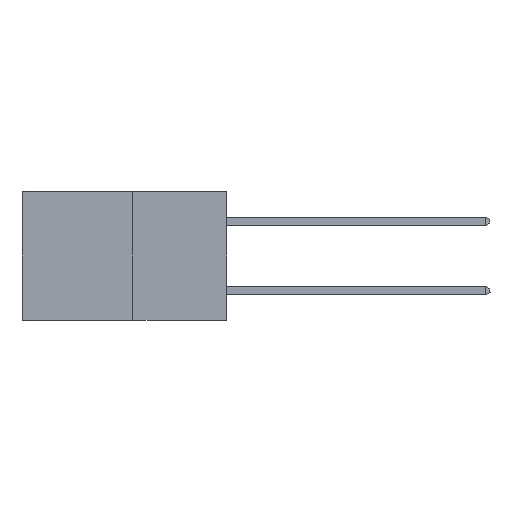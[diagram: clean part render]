
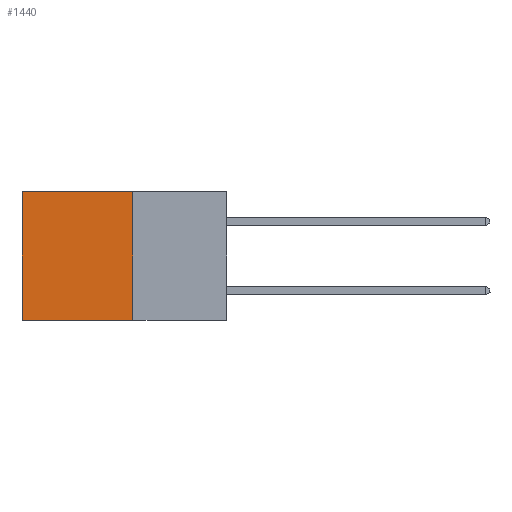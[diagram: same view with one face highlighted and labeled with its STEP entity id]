
A CAD part, left-side view. The second image highlights one B-rep face of the part: STEP entity #1440.
In plain terms, the highlighted planar face has unit normal (-1, 0, 0).
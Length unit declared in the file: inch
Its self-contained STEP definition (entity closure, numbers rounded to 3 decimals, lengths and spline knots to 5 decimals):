
#125 = ORIENTED_EDGE ( 'NONE', *, *, #4721, .T. ) ;
#273 = ORIENTED_EDGE ( 'NONE', *, *, #5878, .F. ) ;
#438 = VERTEX_POINT ( 'NONE', #6912 ) ;
#564 = DIRECTION ( 'NONE',  ( 0., 1., 0. ) ) ;
#742 = CARTESIAN_POINT ( 'NONE',  ( 0.277, 0.27, -0.37 ) ) ;
#805 = LINE ( 'NONE', #8846, #3185 ) ;
#1440 = ADVANCED_FACE ( 'NONE', ( #3838 ), #8367, .F. ) ;
#1533 = CARTESIAN_POINT ( 'NONE',  ( 0.277, 0.59, 0. ) ) ;
#1678 = VERTEX_POINT ( 'NONE', #8122 ) ;
#2023 = VECTOR ( 'NONE', #5683, 39.37008 ) ;
#2305 = LINE ( 'NONE', #2993, #2023 ) ;
#2418 = VECTOR ( 'NONE', #3677, 39.37008 ) ;
#2883 = EDGE_LOOP ( 'NONE', ( #5859, #273, #5127, #125 ) ) ;
#2993 = CARTESIAN_POINT ( 'NONE',  ( 0.277, 0.27, 0. ) ) ;
#3185 = VECTOR ( 'NONE', #564, 39.37008 ) ;
#3573 = DIRECTION ( 'NONE',  ( 0., 0., -1. ) ) ;
#3677 = DIRECTION ( 'NONE',  ( 0., 0., -1. ) ) ;
#3838 = FACE_OUTER_BOUND ( 'NONE', #2883, .T. ) ;
#4116 = LINE ( 'NONE', #9818, #8060 ) ;
#4721 = EDGE_CURVE ( 'NONE', #438, #7566, #2305, .T. ) ;
#4774 = LINE ( 'NONE', #742, #2418 ) ;
#4992 = EDGE_CURVE ( 'NONE', #7566, #9411, #4116, .T. ) ;
#5127 = ORIENTED_EDGE ( 'NONE', *, *, #5328, .F. ) ;
#5328 = EDGE_CURVE ( 'NONE', #438, #1678, #4774, .T. ) ;
#5683 = DIRECTION ( 'NONE',  ( 0., 1., 0. ) ) ;
#5859 = ORIENTED_EDGE ( 'NONE', *, *, #4992, .T. ) ;
#5878 = EDGE_CURVE ( 'NONE', #1678, #9411, #805, .T. ) ;
#6912 = CARTESIAN_POINT ( 'NONE',  ( 0.277, 0.27, 0. ) ) ;
#7566 = VERTEX_POINT ( 'NONE', #1533 ) ;
#8060 = VECTOR ( 'NONE', #3573, 39.37008 ) ;
#8122 = CARTESIAN_POINT ( 'NONE',  ( 0.277, 0.27, -0.37 ) ) ;
#8270 = AXIS2_PLACEMENT_3D ( 'NONE', #8798, #8354, #8316 ) ;
#8316 = DIRECTION ( 'NONE',  ( 0., 0., -1. ) ) ;
#8354 = DIRECTION ( 'NONE',  ( 1., 0., 0. ) ) ;
#8367 = PLANE ( 'NONE',  #8270 ) ;
#8516 = CARTESIAN_POINT ( 'NONE',  ( 0.277, 0.59, -0.37 ) ) ;
#8798 = CARTESIAN_POINT ( 'NONE',  ( 0.277, 0.27, -0.37 ) ) ;
#8846 = CARTESIAN_POINT ( 'NONE',  ( 0.277, 0.27, -0.37 ) ) ;
#9411 = VERTEX_POINT ( 'NONE', #8516 ) ;
#9818 = CARTESIAN_POINT ( 'NONE',  ( 0.277, 0.59, -0.37 ) ) ;
